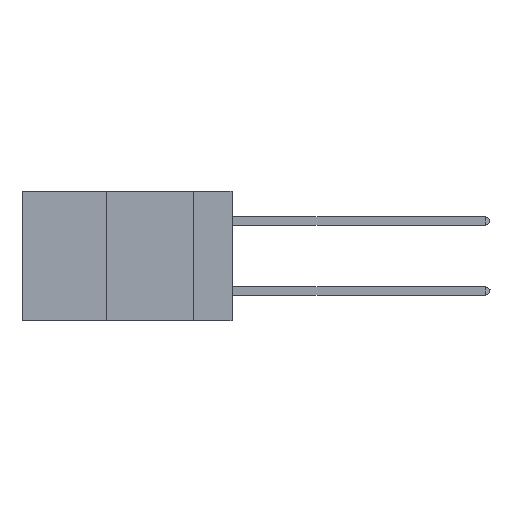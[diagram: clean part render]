
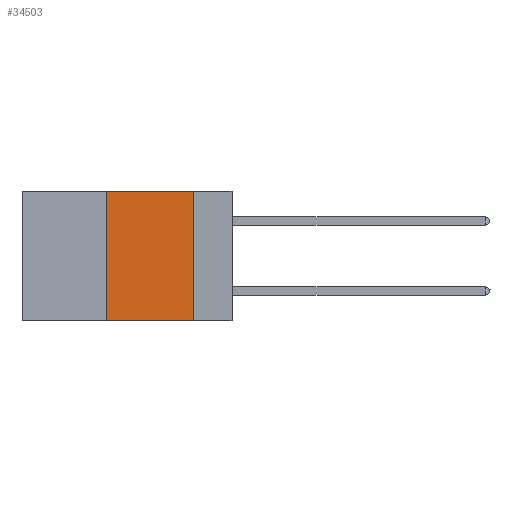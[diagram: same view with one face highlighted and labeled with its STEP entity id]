
A CAD part, left-side view. The second image highlights one B-rep face of the part: STEP entity #34503.
In plain terms, the highlighted planar face has unit normal (-1, 0, 0).
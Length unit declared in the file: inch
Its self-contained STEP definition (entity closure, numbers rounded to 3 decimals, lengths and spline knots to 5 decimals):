
#48 = LINE ( 'NONE', #26292, #32705 ) ;
#1060 = LINE ( 'NONE', #24571, #10908 ) ;
#3480 = EDGE_LOOP ( 'NONE', ( #36224, #25396, #25803, #36088 ) ) ;
#3881 = PLANE ( 'NONE',  #13136 ) ;
#4379 = CARTESIAN_POINT ( 'NONE',  ( 0., 0.36, 0. ) ) ;
#10242 = DIRECTION ( 'NONE',  ( 0., 0., -1. ) ) ;
#10422 = CARTESIAN_POINT ( 'NONE',  ( 0., 0.6, 0. ) ) ;
#10908 = VECTOR ( 'NONE', #33476, 39.37008 ) ;
#11450 = DIRECTION ( 'NONE',  ( 0., 0., 1. ) ) ;
#13136 = AXIS2_PLACEMENT_3D ( 'NONE', #10422, #22012, #10242 ) ;
#13165 = EDGE_CURVE ( 'NONE', #27222, #26667, #1060, .T. ) ;
#14020 = VERTEX_POINT ( 'NONE', #4379 ) ;
#15254 = LINE ( 'NONE', #33032, #23470 ) ;
#15836 = FACE_OUTER_BOUND ( 'NONE', #3480, .T. ) ;
#19245 = EDGE_CURVE ( 'NONE', #27222, #14020, #48, .T. ) ;
#20255 = CARTESIAN_POINT ( 'NONE',  ( 0., 0.11, 0. ) ) ;
#20453 = CARTESIAN_POINT ( 'NONE',  ( 0., 0.6, 0. ) ) ;
#22012 = DIRECTION ( 'NONE',  ( 1., 0., 0. ) ) ;
#23001 = LINE ( 'NONE', #20453, #24056 ) ;
#23327 = CARTESIAN_POINT ( 'NONE',  ( 0., 0.36, -0.37 ) ) ;
#23470 = VECTOR ( 'NONE', #27431, 39.37008 ) ;
#24056 = VECTOR ( 'NONE', #26442, 39.37008 ) ;
#24571 = CARTESIAN_POINT ( 'NONE',  ( 0., 0.6, -0.37 ) ) ;
#25121 = CARTESIAN_POINT ( 'NONE',  ( 0., 0.11, -0.37 ) ) ;
#25396 = ORIENTED_EDGE ( 'NONE', *, *, #30300, .F. ) ;
#25803 = ORIENTED_EDGE ( 'NONE', *, *, #19245, .F. ) ;
#26292 = CARTESIAN_POINT ( 'NONE',  ( 0., 0.36, 0. ) ) ;
#26442 = DIRECTION ( 'NONE',  ( 0., -1., 0. ) ) ;
#26667 = VERTEX_POINT ( 'NONE', #25121 ) ;
#27222 = VERTEX_POINT ( 'NONE', #23327 ) ;
#27431 = DIRECTION ( 'NONE',  ( 0., 0., -1. ) ) ;
#29923 = EDGE_CURVE ( 'NONE', #30229, #26667, #15254, .T. ) ;
#30229 = VERTEX_POINT ( 'NONE', #20255 ) ;
#30300 = EDGE_CURVE ( 'NONE', #14020, #30229, #23001, .T. ) ;
#32705 = VECTOR ( 'NONE', #11450, 39.37008 ) ;
#33032 = CARTESIAN_POINT ( 'NONE',  ( 0., 0.11, 0. ) ) ;
#33476 = DIRECTION ( 'NONE',  ( 0., -1., 0. ) ) ;
#34503 = ADVANCED_FACE ( 'NONE', ( #15836 ), #3881, .F. ) ;
#36088 = ORIENTED_EDGE ( 'NONE', *, *, #13165, .T. ) ;
#36224 = ORIENTED_EDGE ( 'NONE', *, *, #29923, .F. ) ;
